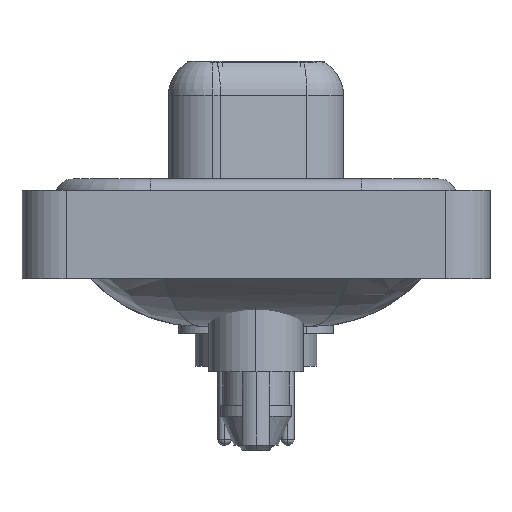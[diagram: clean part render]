
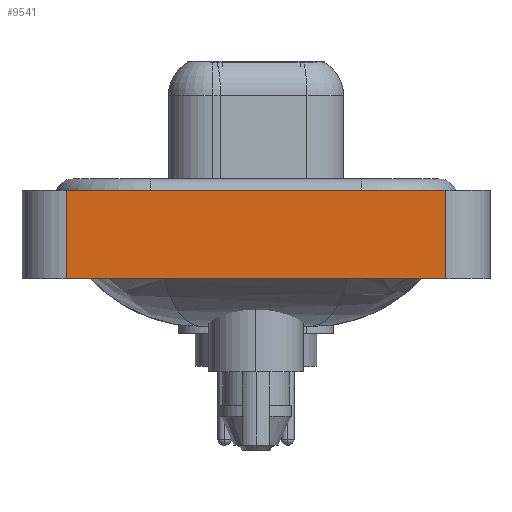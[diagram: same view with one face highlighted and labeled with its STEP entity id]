
A CAD part, left-side view. The second image highlights one B-rep face of the part: STEP entity #9541.
In plain terms, the highlighted planar face has unit normal (-1, 0, 0).
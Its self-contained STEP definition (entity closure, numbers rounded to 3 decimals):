
#223 = PLANE ( 'NONE',  #10161 ) ;
#601 = ORIENTED_EDGE ( 'NONE', *, *, #18523, .F. ) ;
#1273 = CARTESIAN_POINT ( 'NONE',  ( -7.35, -8.55, 0.4 ) ) ;
#2458 = EDGE_CURVE ( 'NONE', #12067, #18642, #21563, .T. ) ;
#3070 = VERTEX_POINT ( 'NONE', #19649 ) ;
#3925 = ORIENTED_EDGE ( 'NONE', *, *, #18785, .F. ) ;
#6172 = EDGE_LOOP ( 'NONE', ( #8458, #3925, #601, #17156 ) ) ;
#6654 = CARTESIAN_POINT ( 'NONE',  ( -7.35, -8.55, -3.6 ) ) ;
#6980 = CARTESIAN_POINT ( 'NONE',  ( -7.35, -8.55, -3.6 ) ) ;
#7774 = EDGE_CURVE ( 'NONE', #18642, #13177, #11984, .T. ) ;
#8045 = VECTOR ( 'NONE', #18345, 1000. ) ;
#8458 = ORIENTED_EDGE ( 'NONE', *, *, #7774, .T. ) ;
#8502 = DIRECTION ( 'NONE',  ( 0., -1., 0. ) ) ;
#9253 = LINE ( 'NONE', #15604, #20276 ) ;
#9541 = ADVANCED_FACE ( 'NONE', ( #20474 ), #223, .T. ) ;
#10161 = AXIS2_PLACEMENT_3D ( 'NONE', #6980, #12112, #10585 ) ;
#10585 = DIRECTION ( 'NONE',  ( 0., 0., 1. ) ) ;
#11662 = DIRECTION ( 'NONE',  ( 0., 0., 1. ) ) ;
#11984 = LINE ( 'NONE', #20016, #13222 ) ;
#12067 = VERTEX_POINT ( 'NONE', #19523 ) ;
#12112 = DIRECTION ( 'NONE',  ( -1., 0., 0. ) ) ;
#13177 = VERTEX_POINT ( 'NONE', #1273 ) ;
#13222 = VECTOR ( 'NONE', #11662, 1000. ) ;
#13299 = LINE ( 'NONE', #18238, #8045 ) ;
#15604 = CARTESIAN_POINT ( 'NONE',  ( -7.35, 8.55, -3.6 ) ) ;
#15928 = DIRECTION ( 'NONE',  ( 0., 0., 1. ) ) ;
#16036 = CARTESIAN_POINT ( 'NONE',  ( -7.35, -8.55, -3.6 ) ) ;
#16943 = VECTOR ( 'NONE', #8502, 1000. ) ;
#17156 = ORIENTED_EDGE ( 'NONE', *, *, #2458, .T. ) ;
#18238 = CARTESIAN_POINT ( 'NONE',  ( -7.35, -8.55, 0.4 ) ) ;
#18345 = DIRECTION ( 'NONE',  ( 0., -1., 0. ) ) ;
#18523 = EDGE_CURVE ( 'NONE', #12067, #3070, #9253, .T. ) ;
#18642 = VERTEX_POINT ( 'NONE', #16036 ) ;
#18785 = EDGE_CURVE ( 'NONE', #3070, #13177, #13299, .T. ) ;
#19523 = CARTESIAN_POINT ( 'NONE',  ( -7.35, 8.55, -3.6 ) ) ;
#19649 = CARTESIAN_POINT ( 'NONE',  ( -7.35, 8.55, 0.4 ) ) ;
#20016 = CARTESIAN_POINT ( 'NONE',  ( -7.35, -8.55, -3.6 ) ) ;
#20276 = VECTOR ( 'NONE', #15928, 1000. ) ;
#20474 = FACE_OUTER_BOUND ( 'NONE', #6172, .T. ) ;
#21563 = LINE ( 'NONE', #6654, #16943 ) ;
